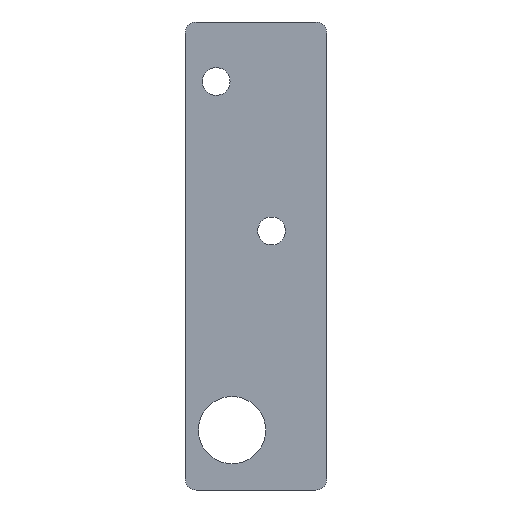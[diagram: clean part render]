
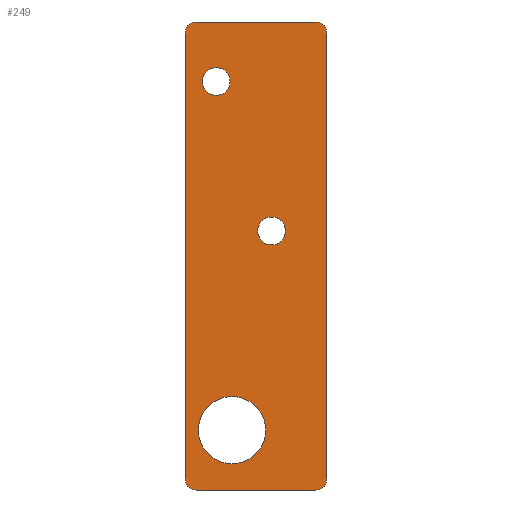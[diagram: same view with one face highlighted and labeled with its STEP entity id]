
A CAD part, left-side view. The second image highlights one B-rep face of the part: STEP entity #249.
In plain terms, the highlighted planar face has unit normal (-1, 0, 0).
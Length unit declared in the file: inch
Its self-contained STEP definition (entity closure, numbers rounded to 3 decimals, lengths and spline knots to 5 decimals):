
#18=FACE_BOUND('',#54,.T.);
#19=FACE_BOUND('',#55,.T.);
#20=FACE_BOUND('',#56,.T.);
#24=PLANE('',#290);
#37=FACE_OUTER_BOUND('',#53,.T.);
#53=EDGE_LOOP('',(#213,#214,#215,#216,#217,#218,#219,#220));
#54=EDGE_LOOP('',(#221));
#55=EDGE_LOOP('',(#222));
#56=EDGE_LOOP('',(#223));
#65=LINE('',#400,#84);
#70=LINE('',#414,#89);
#76=LINE('',#433,#95);
#77=LINE('',#434,#96);
#84=VECTOR('',#323,0.3937);
#89=VECTOR('',#338,0.3937);
#95=VECTOR('',#362,0.3937);
#96=VECTOR('',#363,0.3937);
#97=CIRCLE('',#267,0.0625);
#105=CIRCLE('',#278,0.0625);
#106=CIRCLE('',#280,0.0625);
#107=CIRCLE('',#283,0.0625);
#108=CIRCLE('',#285,0.19);
#109=CIRCLE('',#287,0.07865);
#110=CIRCLE('',#289,0.07865);
#111=VERTEX_POINT('',#370);
#112=VERTEX_POINT('',#371);
#124=VERTEX_POINT('',#399);
#125=VERTEX_POINT('',#403);
#126=VERTEX_POINT('',#407);
#127=VERTEX_POINT('',#409);
#128=VERTEX_POINT('',#413);
#129=VERTEX_POINT('',#417);
#130=VERTEX_POINT('',#421);
#131=VERTEX_POINT('',#425);
#132=VERTEX_POINT('',#429);
#133=EDGE_CURVE('',#111,#112,#97,.T.);
#147=EDGE_CURVE('',#112,#124,#65,.T.);
#149=EDGE_CURVE('',#124,#125,#105,.T.);
#152=EDGE_CURVE('',#126,#127,#106,.T.);
#154=EDGE_CURVE('',#128,#127,#70,.F.);
#156=EDGE_CURVE('',#128,#129,#107,.T.);
#159=EDGE_CURVE('',#130,#130,#108,.T.);
#161=EDGE_CURVE('',#131,#131,#109,.T.);
#163=EDGE_CURVE('',#132,#132,#110,.T.);
#164=EDGE_CURVE('',#111,#129,#76,.T.);
#165=EDGE_CURVE('',#125,#126,#77,.F.);
#213=ORIENTED_EDGE('',*,*,#133,.F.);
#214=ORIENTED_EDGE('',*,*,#164,.T.);
#215=ORIENTED_EDGE('',*,*,#156,.F.);
#216=ORIENTED_EDGE('',*,*,#154,.T.);
#217=ORIENTED_EDGE('',*,*,#152,.F.);
#218=ORIENTED_EDGE('',*,*,#165,.F.);
#219=ORIENTED_EDGE('',*,*,#149,.F.);
#220=ORIENTED_EDGE('',*,*,#147,.F.);
#221=ORIENTED_EDGE('',*,*,#159,.T.);
#222=ORIENTED_EDGE('',*,*,#161,.T.);
#223=ORIENTED_EDGE('',*,*,#163,.T.);
#249=ADVANCED_FACE('',(#37,#18,#19,#20),#24,.T.);
#267=AXIS2_PLACEMENT_3D('',#372,#297,#298);
#278=AXIS2_PLACEMENT_3D('',#404,#327,#328);
#280=AXIS2_PLACEMENT_3D('',#410,#333,#334);
#283=AXIS2_PLACEMENT_3D('',#418,#342,#343);
#285=AXIS2_PLACEMENT_3D('',#423,#348,#349);
#287=AXIS2_PLACEMENT_3D('',#427,#353,#354);
#289=AXIS2_PLACEMENT_3D('',#431,#358,#359);
#290=AXIS2_PLACEMENT_3D('',#432,#360,#361);
#297=DIRECTION('center_axis',(1.,0.,0.));
#298=DIRECTION('ref_axis',(0.,0.707,0.707));
#323=DIRECTION('',(0.,-1.,0.));
#327=DIRECTION('center_axis',(1.,0.,0.));
#328=DIRECTION('ref_axis',(0.,-0.707,0.707));
#333=DIRECTION('center_axis',(1.,0.,0.));
#334=DIRECTION('ref_axis',(0.,-0.707,-0.707));
#338=DIRECTION('',(0.,1.,0.));
#342=DIRECTION('center_axis',(1.,0.,0.));
#343=DIRECTION('ref_axis',(0.,0.707,-0.707));
#348=DIRECTION('center_axis',(1.,0.,0.));
#349=DIRECTION('ref_axis',(0.,0.,-1.));
#353=DIRECTION('center_axis',(1.,0.,0.));
#354=DIRECTION('ref_axis',(0.,0.,-1.));
#358=DIRECTION('center_axis',(1.,0.,0.));
#359=DIRECTION('ref_axis',(0.,0.,-1.));
#360=DIRECTION('center_axis',(-1.,0.,0.));
#361=DIRECTION('ref_axis',(0.,0.,-1.));
#362=DIRECTION('',(0.,0.,-1.));
#363=DIRECTION('',(0.,0.,1.));
#370=CARTESIAN_POINT('',(0.3475,-0.45,-0.06644));
#371=CARTESIAN_POINT('',(0.3475,-0.5125,-0.00394));
#372=CARTESIAN_POINT('Origin',(0.3475,-0.5125,-0.06644));
#399=CARTESIAN_POINT('',(0.3475,-1.18756,-0.00394));
#400=CARTESIAN_POINT('',(0.3475,-0.45,-0.00394));
#403=CARTESIAN_POINT('',(0.3475,-1.25006,-0.06644));
#404=CARTESIAN_POINT('Origin',(0.3475,-1.18756,-0.06644));
#407=CARTESIAN_POINT('',(0.3475,-1.25006,-2.58456));
#409=CARTESIAN_POINT('',(0.3475,-1.18756,-2.64706));
#410=CARTESIAN_POINT('Origin',(0.3475,-1.18756,-2.58456));
#413=CARTESIAN_POINT('',(0.3475,-0.5125,-2.64706));
#414=CARTESIAN_POINT('',(0.3475,-0.45,-2.64706));
#417=CARTESIAN_POINT('',(0.3475,-0.45,-2.58456));
#418=CARTESIAN_POINT('Origin',(0.3475,-0.5125,-2.58456));
#421=CARTESIAN_POINT('',(0.3475,-0.715,-2.119));
#423=CARTESIAN_POINT('Origin',(0.3475,-0.715,-2.309));
#425=CARTESIAN_POINT('',(0.3475,-0.938,-1.10535));
#427=CARTESIAN_POINT('Origin',(0.3475,-0.938,-1.184));
#429=CARTESIAN_POINT('',(0.3475,-0.625,-0.26135));
#431=CARTESIAN_POINT('Origin',(0.3475,-0.625,-0.34));
#432=CARTESIAN_POINT('Origin',(0.3475,-0.45,0.));
#433=CARTESIAN_POINT('',(0.3475,-0.45,-0.66275));
#434=CARTESIAN_POINT('',(0.3475,-1.25006,-0.66275));
